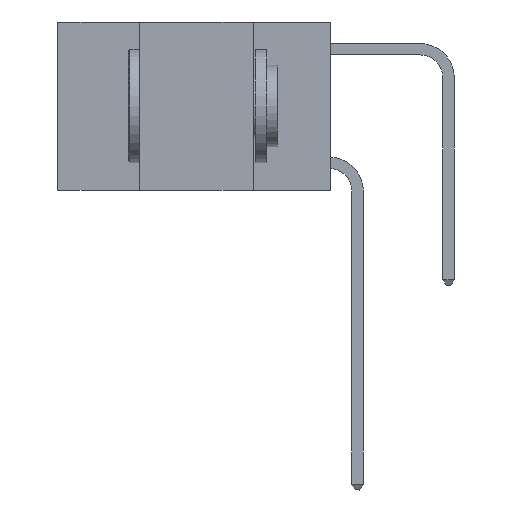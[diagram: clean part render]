
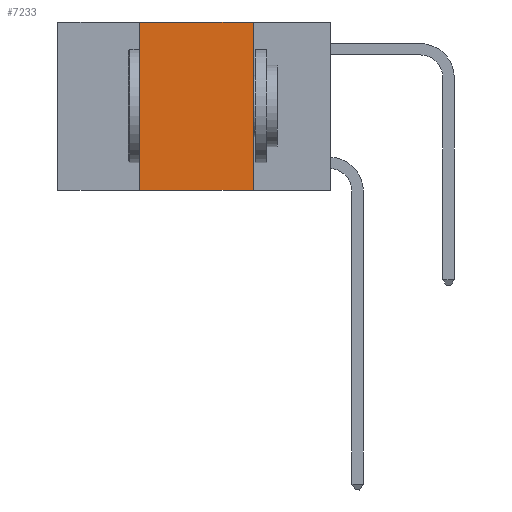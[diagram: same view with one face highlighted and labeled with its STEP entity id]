
A CAD part, left-side view. The second image highlights one B-rep face of the part: STEP entity #7233.
In plain terms, the highlighted planar face has unit normal (-1, 0, 0).
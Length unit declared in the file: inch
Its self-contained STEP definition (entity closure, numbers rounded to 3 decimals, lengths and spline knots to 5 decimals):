
#454 = PLANE ( 'NONE',  #8460 ) ;
#779 = ORIENTED_EDGE ( 'NONE', *, *, #3257, .F. ) ;
#819 = VERTEX_POINT ( 'NONE', #3456 ) ;
#1588 = VECTOR ( 'NONE', #6919, 39.37008 ) ;
#2027 = CARTESIAN_POINT ( 'NONE',  ( 0., 0.42, 0. ) ) ;
#2072 = ORIENTED_EDGE ( 'NONE', *, *, #3360, .F. ) ;
#2251 = DIRECTION ( 'NONE',  ( 0., 0., -1. ) ) ;
#2853 = LINE ( 'NONE', #8227, #9468 ) ;
#3130 = LINE ( 'NONE', #6849, #5220 ) ;
#3209 = ORIENTED_EDGE ( 'NONE', *, *, #3397, .T. ) ;
#3257 = EDGE_CURVE ( 'NONE', #819, #8046, #3990, .T. ) ;
#3360 = EDGE_CURVE ( 'NONE', #4358, #819, #3130, .T. ) ;
#3397 = EDGE_CURVE ( 'NONE', #4092, #8046, #2853, .T. ) ;
#3456 = CARTESIAN_POINT ( 'NONE',  ( 0., 0.17, 0. ) ) ;
#3990 = LINE ( 'NONE', #4196, #1588 ) ;
#4092 = VERTEX_POINT ( 'NONE', #4820 ) ;
#4144 = VECTOR ( 'NONE', #8883, 39.37008 ) ;
#4196 = CARTESIAN_POINT ( 'NONE',  ( 0., 0.17, 0. ) ) ;
#4326 = CARTESIAN_POINT ( 'NONE',  ( 0., 0.17, -0.37 ) ) ;
#4358 = VERTEX_POINT ( 'NONE', #11142 ) ;
#4820 = CARTESIAN_POINT ( 'NONE',  ( 0., 0.42, -0.37 ) ) ;
#5220 = VECTOR ( 'NONE', #5688, 39.37008 ) ;
#5236 = ORIENTED_EDGE ( 'NONE', *, *, #8385, .F. ) ;
#5688 = DIRECTION ( 'NONE',  ( 0., -1., 0. ) ) ;
#6849 = CARTESIAN_POINT ( 'NONE',  ( 0., 0.6, 0. ) ) ;
#6919 = DIRECTION ( 'NONE',  ( 0., 0., -1. ) ) ;
#7233 = ADVANCED_FACE ( 'NONE', ( #9644 ), #454, .F. ) ;
#7481 = DIRECTION ( 'NONE',  ( 1., 0., 0. ) ) ;
#8046 = VERTEX_POINT ( 'NONE', #4326 ) ;
#8227 = CARTESIAN_POINT ( 'NONE',  ( 0., 0.6, -0.37 ) ) ;
#8385 = EDGE_CURVE ( 'NONE', #4092, #4358, #8397, .T. ) ;
#8397 = LINE ( 'NONE', #2027, #4144 ) ;
#8460 = AXIS2_PLACEMENT_3D ( 'NONE', #10929, #7481, #2251 ) ;
#8883 = DIRECTION ( 'NONE',  ( 0., 0., 1. ) ) ;
#9110 = EDGE_LOOP ( 'NONE', ( #779, #2072, #5236, #3209 ) ) ;
#9468 = VECTOR ( 'NONE', #11281, 39.37008 ) ;
#9644 = FACE_OUTER_BOUND ( 'NONE', #9110, .T. ) ;
#10929 = CARTESIAN_POINT ( 'NONE',  ( 0., 0.6, 0. ) ) ;
#11142 = CARTESIAN_POINT ( 'NONE',  ( 0., 0.42, 0. ) ) ;
#11281 = DIRECTION ( 'NONE',  ( 0., -1., 0. ) ) ;
